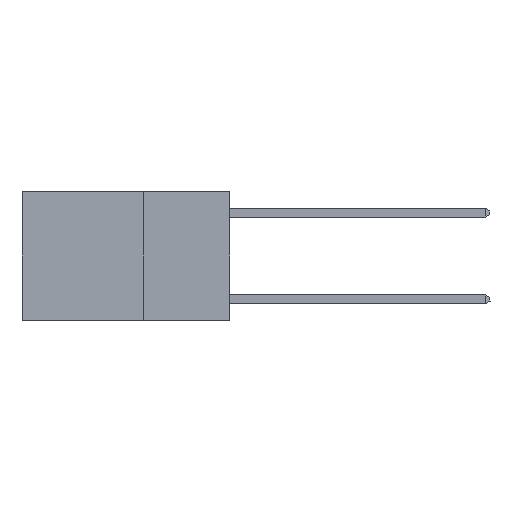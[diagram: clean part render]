
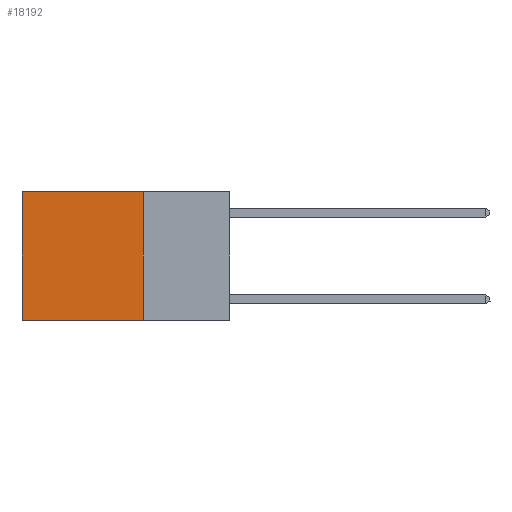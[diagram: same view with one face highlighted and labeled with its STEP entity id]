
A CAD part, left-side view. The second image highlights one B-rep face of the part: STEP entity #18192.
In plain terms, the highlighted planar face has unit normal (-1, 0, 0).
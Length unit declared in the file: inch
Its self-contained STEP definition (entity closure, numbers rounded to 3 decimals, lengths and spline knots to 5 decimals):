
#46 = CARTESIAN_POINT ( 'NONE',  ( 0.2625, 0.6, -0.37 ) ) ;
#931 = LINE ( 'NONE', #2030, #9100 ) ;
#983 = DIRECTION ( 'NONE',  ( 0., 0., -1. ) ) ;
#1511 = VERTEX_POINT ( 'NONE', #46 ) ;
#1651 = CARTESIAN_POINT ( 'NONE',  ( 0.2625, 0.25, 0. ) ) ;
#2030 = CARTESIAN_POINT ( 'NONE',  ( 0.2625, 0.25, 0. ) ) ;
#2369 = VECTOR ( 'NONE', #19528, 39.37008 ) ;
#2569 = LINE ( 'NONE', #8536, #10332 ) ;
#2650 = DIRECTION ( 'NONE',  ( 1., 0., 0. ) ) ;
#2719 = VERTEX_POINT ( 'NONE', #5240 ) ;
#2927 = VECTOR ( 'NONE', #3752, 39.37008 ) ;
#3752 = DIRECTION ( 'NONE',  ( 0., 0., -1. ) ) ;
#5240 = CARTESIAN_POINT ( 'NONE',  ( 0.2625, 0.25, -0.37 ) ) ;
#6349 = AXIS2_PLACEMENT_3D ( 'NONE', #10387, #2650, #13460 ) ;
#8536 = CARTESIAN_POINT ( 'NONE',  ( 0.2625, 0.6, 0. ) ) ;
#9100 = VECTOR ( 'NONE', #11279, 39.37008 ) ;
#9597 = EDGE_CURVE ( 'NONE', #18876, #16579, #931, .T. ) ;
#10332 = VECTOR ( 'NONE', #983, 39.37008 ) ;
#10387 = CARTESIAN_POINT ( 'NONE',  ( 0.2625, 0.25, 0. ) ) ;
#10539 = CARTESIAN_POINT ( 'NONE',  ( 0.2625, 0.25, -0.37 ) ) ;
#10611 = LINE ( 'NONE', #10539, #2369 ) ;
#11136 = ORIENTED_EDGE ( 'NONE', *, *, #15362, .F. ) ;
#11139 = EDGE_CURVE ( 'NONE', #16579, #1511, #2569, .T. ) ;
#11279 = DIRECTION ( 'NONE',  ( 0., 1., 0. ) ) ;
#12011 = EDGE_LOOP ( 'NONE', ( #18186, #11136, #15216, #19586 ) ) ;
#12121 = LINE ( 'NONE', #17525, #2927 ) ;
#13460 = DIRECTION ( 'NONE',  ( 0., 0., -1. ) ) ;
#15216 = ORIENTED_EDGE ( 'NONE', *, *, #18014, .F. ) ;
#15362 = EDGE_CURVE ( 'NONE', #2719, #1511, #10611, .T. ) ;
#16429 = PLANE ( 'NONE',  #6349 ) ;
#16579 = VERTEX_POINT ( 'NONE', #19356 ) ;
#16873 = FACE_OUTER_BOUND ( 'NONE', #12011, .T. ) ;
#17525 = CARTESIAN_POINT ( 'NONE',  ( 0.2625, 0.25, 0. ) ) ;
#18014 = EDGE_CURVE ( 'NONE', #18876, #2719, #12121, .T. ) ;
#18186 = ORIENTED_EDGE ( 'NONE', *, *, #11139, .T. ) ;
#18192 = ADVANCED_FACE ( 'NONE', ( #16873 ), #16429, .F. ) ;
#18876 = VERTEX_POINT ( 'NONE', #1651 ) ;
#19356 = CARTESIAN_POINT ( 'NONE',  ( 0.2625, 0.6, 0. ) ) ;
#19528 = DIRECTION ( 'NONE',  ( 0., 1., 0. ) ) ;
#19586 = ORIENTED_EDGE ( 'NONE', *, *, #9597, .T. ) ;
